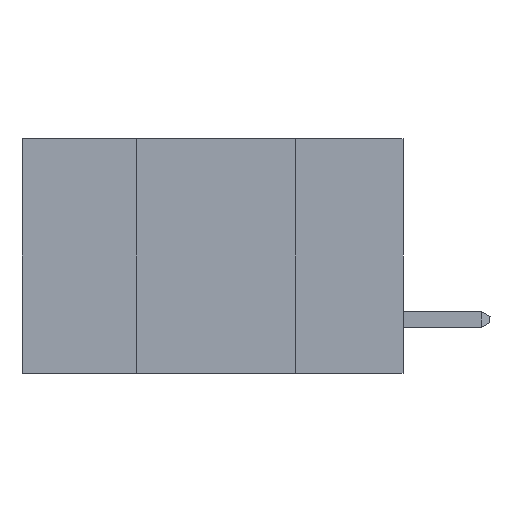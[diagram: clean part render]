
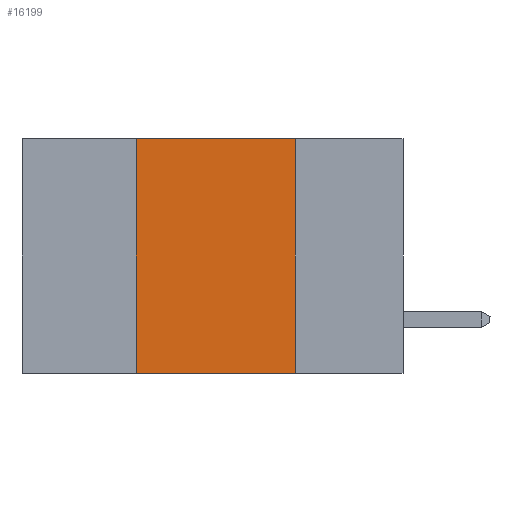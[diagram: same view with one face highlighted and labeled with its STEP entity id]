
A CAD part, left-side view. The second image highlights one B-rep face of the part: STEP entity #16199.
In plain terms, the highlighted planar face has unit normal (-1, 0, 0).
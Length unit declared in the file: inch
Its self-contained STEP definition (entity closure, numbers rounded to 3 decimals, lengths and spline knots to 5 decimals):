
#241 = DIRECTION ( 'NONE',  ( 0., 0., 1. ) ) ;
#1090 = LINE ( 'NONE', #43328, #23635 ) ;
#1627 = VECTOR ( 'NONE', #3270, 39.37008 ) ;
#3270 = DIRECTION ( 'NONE',  ( 0., -1., 0. ) ) ;
#3373 = DIRECTION ( 'NONE',  ( 0., 0., -1. ) ) ;
#4102 = VERTEX_POINT ( 'NONE', #13908 ) ;
#4561 = ORIENTED_EDGE ( 'NONE', *, *, #20695, .F. ) ;
#5242 = EDGE_CURVE ( 'NONE', #35242, #28365, #25643, .T. ) ;
#7115 = CARTESIAN_POINT ( 'NONE',  ( 0., 0.42, 0. ) ) ;
#7575 = DIRECTION ( 'NONE',  ( 0., -1., 0. ) ) ;
#8253 = VERTEX_POINT ( 'NONE', #46097 ) ;
#11449 = CARTESIAN_POINT ( 'NONE',  ( 0., 0.42, 0. ) ) ;
#12984 = FACE_OUTER_BOUND ( 'NONE', #34736, .T. ) ;
#13322 = DIRECTION ( 'NONE',  ( 1., 0., 0. ) ) ;
#13908 = CARTESIAN_POINT ( 'NONE',  ( 0., 0.17, 0. ) ) ;
#16199 = ADVANCED_FACE ( 'NONE', ( #12984 ), #24256, .F. ) ;
#18459 = ORIENTED_EDGE ( 'NONE', *, *, #5242, .F. ) ;
#20695 = EDGE_CURVE ( 'NONE', #28365, #4102, #28806, .T. ) ;
#23635 = VECTOR ( 'NONE', #3373, 39.37008 ) ;
#24256 = PLANE ( 'NONE',  #44282 ) ;
#24932 = DIRECTION ( 'NONE',  ( 0., 0., -1. ) ) ;
#25643 = LINE ( 'NONE', #11449, #36563 ) ;
#27371 = EDGE_CURVE ( 'NONE', #4102, #8253, #1090, .T. ) ;
#27816 = ORIENTED_EDGE ( 'NONE', *, *, #32647, .T. ) ;
#28365 = VERTEX_POINT ( 'NONE', #7115 ) ;
#28806 = LINE ( 'NONE', #43545, #1627 ) ;
#29079 = CARTESIAN_POINT ( 'NONE',  ( 0., 0.42, -0.37 ) ) ;
#29082 = CARTESIAN_POINT ( 'NONE',  ( 0., 0.6, -0.37 ) ) ;
#32647 = EDGE_CURVE ( 'NONE', #35242, #8253, #38052, .T. ) ;
#34736 = EDGE_LOOP ( 'NONE', ( #35774, #4561, #18459, #27816 ) ) ;
#35242 = VERTEX_POINT ( 'NONE', #29079 ) ;
#35774 = ORIENTED_EDGE ( 'NONE', *, *, #27371, .F. ) ;
#36563 = VECTOR ( 'NONE', #241, 39.37008 ) ;
#38052 = LINE ( 'NONE', #29082, #44917 ) ;
#43328 = CARTESIAN_POINT ( 'NONE',  ( 0., 0.17, 0. ) ) ;
#43545 = CARTESIAN_POINT ( 'NONE',  ( 0., 0.6, 0. ) ) ;
#44282 = AXIS2_PLACEMENT_3D ( 'NONE', #46767, #13322, #24932 ) ;
#44917 = VECTOR ( 'NONE', #7575, 39.37008 ) ;
#46097 = CARTESIAN_POINT ( 'NONE',  ( 0., 0.17, -0.37 ) ) ;
#46767 = CARTESIAN_POINT ( 'NONE',  ( 0., 0.6, 0. ) ) ;
